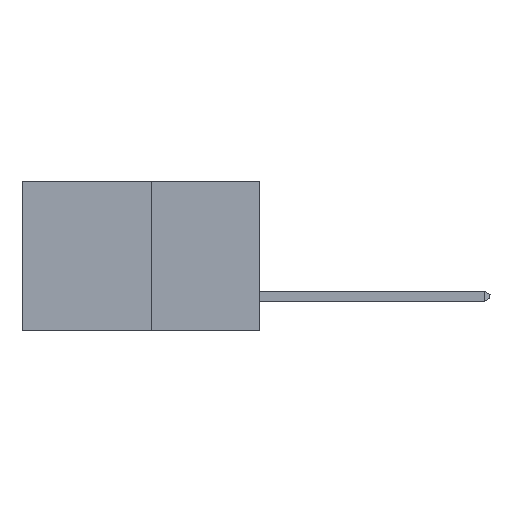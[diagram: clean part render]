
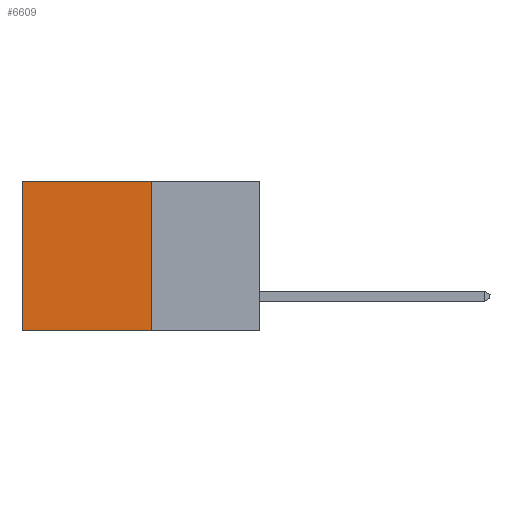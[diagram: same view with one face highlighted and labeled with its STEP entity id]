
A CAD part, left-side view. The second image highlights one B-rep face of the part: STEP entity #6609.
In plain terms, the highlighted planar face has unit normal (-1, 0, 0).
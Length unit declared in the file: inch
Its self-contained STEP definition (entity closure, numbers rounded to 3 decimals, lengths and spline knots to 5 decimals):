
#422 = VERTEX_POINT ( 'NONE', #1089 ) ;
#436 = VECTOR ( 'NONE', #1091, 39.37008 ) ;
#573 = EDGE_CURVE ( 'NONE', #10284, #1686, #10353, .T. ) ;
#1089 = CARTESIAN_POINT ( 'NONE',  ( 0.277, 0.59, 0. ) ) ;
#1091 = DIRECTION ( 'NONE',  ( 0., 1., 0. ) ) ;
#1123 = CARTESIAN_POINT ( 'NONE',  ( 0.277, 0.27, 0. ) ) ;
#1144 = CARTESIAN_POINT ( 'NONE',  ( 0.277, 0.27, -0.37 ) ) ;
#1348 = DIRECTION ( 'NONE',  ( 0., 0., -1. ) ) ;
#1686 = VERTEX_POINT ( 'NONE', #8491 ) ;
#1862 = CARTESIAN_POINT ( 'NONE',  ( 0.277, 0.27, 0. ) ) ;
#1940 = FACE_OUTER_BOUND ( 'NONE', #11055, .T. ) ;
#2011 = EDGE_CURVE ( 'NONE', #422, #7754, #6476, .T. ) ;
#2448 = ORIENTED_EDGE ( 'NONE', *, *, #2011, .T. ) ;
#3133 = ORIENTED_EDGE ( 'NONE', *, *, #7186, .F. ) ;
#3675 = VECTOR ( 'NONE', #6973, 39.37008 ) ;
#4663 = DIRECTION ( 'NONE',  ( 0., 1., 0. ) ) ;
#4801 = EDGE_CURVE ( 'NONE', #10284, #422, #5871, .T. ) ;
#4817 = VECTOR ( 'NONE', #8639, 39.37008 ) ;
#5267 = LINE ( 'NONE', #7803, #5933 ) ;
#5351 = ORIENTED_EDGE ( 'NONE', *, *, #4801, .T. ) ;
#5871 = LINE ( 'NONE', #1123, #436 ) ;
#5933 = VECTOR ( 'NONE', #4663, 39.37008 ) ;
#6476 = LINE ( 'NONE', #10152, #3675 ) ;
#6609 = ADVANCED_FACE ( 'NONE', ( #1940 ), #12831, .F. ) ;
#6699 = CARTESIAN_POINT ( 'NONE',  ( 0.277, 0.27, -0.37 ) ) ;
#6973 = DIRECTION ( 'NONE',  ( 0., 0., -1. ) ) ;
#7186 = EDGE_CURVE ( 'NONE', #1686, #7754, #5267, .T. ) ;
#7463 = CARTESIAN_POINT ( 'NONE',  ( 0.277, 0.59, -0.37 ) ) ;
#7754 = VERTEX_POINT ( 'NONE', #7463 ) ;
#7766 = DIRECTION ( 'NONE',  ( 1., 0., 0. ) ) ;
#7803 = CARTESIAN_POINT ( 'NONE',  ( 0.277, 0.27, -0.37 ) ) ;
#8491 = CARTESIAN_POINT ( 'NONE',  ( 0.277, 0.27, -0.37 ) ) ;
#8639 = DIRECTION ( 'NONE',  ( 0., 0., -1. ) ) ;
#9744 = AXIS2_PLACEMENT_3D ( 'NONE', #6699, #7766, #1348 ) ;
#10152 = CARTESIAN_POINT ( 'NONE',  ( 0.277, 0.59, -0.37 ) ) ;
#10284 = VERTEX_POINT ( 'NONE', #1862 ) ;
#10353 = LINE ( 'NONE', #1144, #4817 ) ;
#11055 = EDGE_LOOP ( 'NONE', ( #2448, #3133, #12648, #5351 ) ) ;
#12648 = ORIENTED_EDGE ( 'NONE', *, *, #573, .F. ) ;
#12831 = PLANE ( 'NONE',  #9744 ) ;
